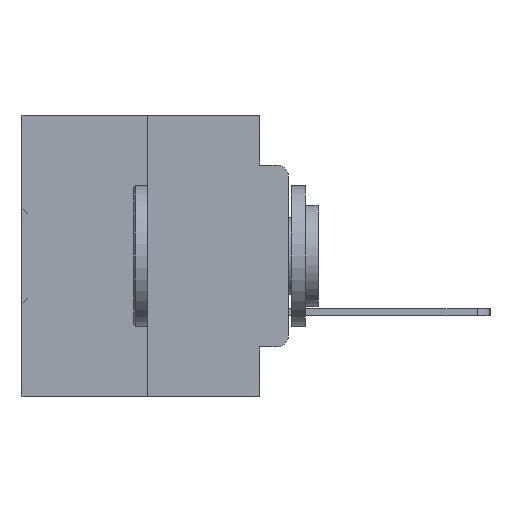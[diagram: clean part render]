
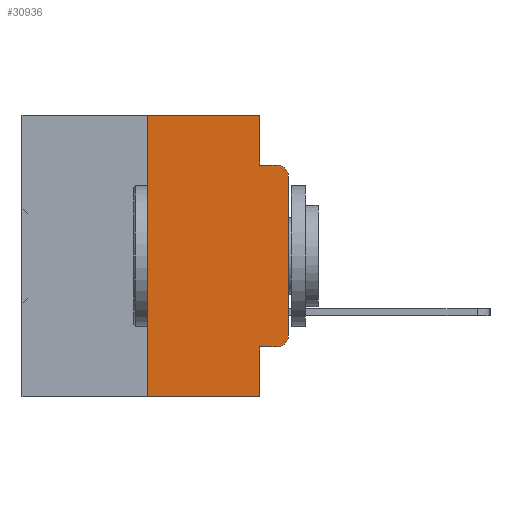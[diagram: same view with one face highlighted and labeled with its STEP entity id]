
A CAD part, left-side view. The second image highlights one B-rep face of the part: STEP entity #30936.
In plain terms, the highlighted planar face has unit normal (-1, 0, 0).
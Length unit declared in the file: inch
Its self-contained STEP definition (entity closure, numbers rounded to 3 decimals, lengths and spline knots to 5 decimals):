
#434 = EDGE_CURVE ( 'NONE', #21544, #3666, #11660, .T. ) ;
#858 = LINE ( 'NONE', #2603, #28845 ) ;
#1403 = DIRECTION ( 'NONE',  ( 0., -1., 0. ) ) ;
#2603 = CARTESIAN_POINT ( 'NONE',  ( 0., 0.051, 0. ) ) ;
#3363 = VECTOR ( 'NONE', #6570, 39.37008 ) ;
#3666 = VERTEX_POINT ( 'NONE', #14622 ) ;
#3934 = CARTESIAN_POINT ( 'NONE',  ( 0., 0.02, -0.4115 ) ) ;
#4176 = ORIENTED_EDGE ( 'NONE', *, *, #11618, .T. ) ;
#4293 = CARTESIAN_POINT ( 'NONE',  ( 0., 0.25, 0. ) ) ;
#4491 = DIRECTION ( 'NONE',  ( 0., 0., 1. ) ) ;
#4858 = DIRECTION ( 'NONE',  ( 0., 0., -1. ) ) ;
#5306 = CARTESIAN_POINT ( 'NONE',  ( 0., 0.051, -0.5 ) ) ;
#6570 = DIRECTION ( 'NONE',  ( 0., 0., 1. ) ) ;
#7183 = LINE ( 'NONE', #12936, #22173 ) ;
#7566 = LINE ( 'NONE', #7788, #21668 ) ;
#7788 = CARTESIAN_POINT ( 'NONE',  ( 0., 0.051, -0.0885 ) ) ;
#7818 = CARTESIAN_POINT ( 'NONE',  ( 0., 0.051, 0. ) ) ;
#8571 = LINE ( 'NONE', #11270, #30840 ) ;
#9204 = VERTEX_POINT ( 'NONE', #5306 ) ;
#9819 = DIRECTION ( 'NONE',  ( -1., 0., 0. ) ) ;
#9824 = EDGE_CURVE ( 'NONE', #34088, #9204, #858, .T. ) ;
#10353 = AXIS2_PLACEMENT_3D ( 'NONE', #26600, #9819, #29366 ) ;
#10611 = DIRECTION ( 'NONE',  ( 0., -1., 0. ) ) ;
#11270 = CARTESIAN_POINT ( 'NONE',  ( 0., 0.051, -0.4115 ) ) ;
#11326 = EDGE_CURVE ( 'NONE', #3666, #15768, #35539, .T. ) ;
#11618 = EDGE_CURVE ( 'NONE', #21544, #9204, #33386, .T. ) ;
#11660 = LINE ( 'NONE', #4293, #3363 ) ;
#11675 = EDGE_CURVE ( 'NONE', #34088, #20534, #8571, .T. ) ;
#12374 = EDGE_CURVE ( 'NONE', #32485, #26978, #7183, .T. ) ;
#12926 = VERTEX_POINT ( 'NONE', #15897 ) ;
#12936 = CARTESIAN_POINT ( 'NONE',  ( 0., 0., 0. ) ) ;
#12945 = DIRECTION ( 'NONE',  ( -1., 0., 0. ) ) ;
#14622 = CARTESIAN_POINT ( 'NONE',  ( 0., 0.25, 0. ) ) ;
#15768 = VERTEX_POINT ( 'NONE', #19610 ) ;
#15897 = CARTESIAN_POINT ( 'NONE',  ( 0., 0.051, -0.0885 ) ) ;
#16616 = CARTESIAN_POINT ( 'NONE',  ( 0., 0., -0.3915 ) ) ;
#17797 = LINE ( 'NONE', #7818, #33356 ) ;
#18198 = CARTESIAN_POINT ( 'NONE',  ( 0., 0.473, 0. ) ) ;
#18888 = CARTESIAN_POINT ( 'NONE',  ( 0., 0.473, 0. ) ) ;
#19427 = CARTESIAN_POINT ( 'NONE',  ( 0., 0.473, -0.5 ) ) ;
#19610 = CARTESIAN_POINT ( 'NONE',  ( 0., 0.051, 0. ) ) ;
#20534 = VERTEX_POINT ( 'NONE', #3934 ) ;
#21140 = EDGE_CURVE ( 'NONE', #20534, #32485, #33394, .T. ) ;
#21544 = VERTEX_POINT ( 'NONE', #30998 ) ;
#21668 = VECTOR ( 'NONE', #10611, 39.37008 ) ;
#21682 = AXIS2_PLACEMENT_3D ( 'NONE', #18888, #21716, #4858 ) ;
#21716 = DIRECTION ( 'NONE',  ( 1., 0., 0. ) ) ;
#21848 = EDGE_CURVE ( 'NONE', #26978, #22989, #25652, .T. ) ;
#22038 = CARTESIAN_POINT ( 'NONE',  ( 0., 0.051, -0.4115 ) ) ;
#22173 = VECTOR ( 'NONE', #4491, 39.37008 ) ;
#22989 = VERTEX_POINT ( 'NONE', #25548 ) ;
#23735 = EDGE_CURVE ( 'NONE', #12926, #22989, #7566, .T. ) ;
#24483 = EDGE_LOOP ( 'NONE', ( #26079, #26947, #35911, #29550, #31238, #24814, #4176, #26537, #34633, #35496 ) ) ;
#24814 = ORIENTED_EDGE ( 'NONE', *, *, #434, .F. ) ;
#25254 = CARTESIAN_POINT ( 'NONE',  ( 0., 0., -0.1085 ) ) ;
#25268 = VECTOR ( 'NONE', #35903, 39.37008 ) ;
#25548 = CARTESIAN_POINT ( 'NONE',  ( 0., 0.02, -0.0885 ) ) ;
#25652 = CIRCLE ( 'NONE', #25857, 0.02 ) ;
#25857 = AXIS2_PLACEMENT_3D ( 'NONE', #29688, #12945, #32399 ) ;
#26079 = ORIENTED_EDGE ( 'NONE', *, *, #12374, .T. ) ;
#26537 = ORIENTED_EDGE ( 'NONE', *, *, #9824, .F. ) ;
#26600 = CARTESIAN_POINT ( 'NONE',  ( 0., 0.02, -0.3915 ) ) ;
#26947 = ORIENTED_EDGE ( 'NONE', *, *, #21848, .T. ) ;
#26978 = VERTEX_POINT ( 'NONE', #25254 ) ;
#27420 = DIRECTION ( 'NONE',  ( 0., 0., -1. ) ) ;
#27801 = DIRECTION ( 'NONE',  ( 0., 0., -1. ) ) ;
#28845 = VECTOR ( 'NONE', #27801, 39.37008 ) ;
#29161 = VECTOR ( 'NONE', #1403, 39.37008 ) ;
#29366 = DIRECTION ( 'NONE',  ( 0., 0., -1. ) ) ;
#29550 = ORIENTED_EDGE ( 'NONE', *, *, #34700, .F. ) ;
#29688 = CARTESIAN_POINT ( 'NONE',  ( 0., 0.02, -0.1085 ) ) ;
#30009 = FACE_OUTER_BOUND ( 'NONE', #24483, .T. ) ;
#30788 = DIRECTION ( 'NONE',  ( 0., -1., 0. ) ) ;
#30840 = VECTOR ( 'NONE', #30788, 39.37008 ) ;
#30936 = ADVANCED_FACE ( 'NONE', ( #30009 ), #35382, .F. ) ;
#30998 = CARTESIAN_POINT ( 'NONE',  ( 0., 0.25, -0.5 ) ) ;
#31238 = ORIENTED_EDGE ( 'NONE', *, *, #11326, .F. ) ;
#32399 = DIRECTION ( 'NONE',  ( 0., 0., -1. ) ) ;
#32485 = VERTEX_POINT ( 'NONE', #16616 ) ;
#33356 = VECTOR ( 'NONE', #27420, 39.37008 ) ;
#33386 = LINE ( 'NONE', #19427, #25268 ) ;
#33394 = CIRCLE ( 'NONE', #10353, 0.02 ) ;
#34088 = VERTEX_POINT ( 'NONE', #22038 ) ;
#34633 = ORIENTED_EDGE ( 'NONE', *, *, #11675, .T. ) ;
#34700 = EDGE_CURVE ( 'NONE', #15768, #12926, #17797, .T. ) ;
#35382 = PLANE ( 'NONE',  #21682 ) ;
#35496 = ORIENTED_EDGE ( 'NONE', *, *, #21140, .T. ) ;
#35539 = LINE ( 'NONE', #18198, #29161 ) ;
#35903 = DIRECTION ( 'NONE',  ( 0., -1., 0. ) ) ;
#35911 = ORIENTED_EDGE ( 'NONE', *, *, #23735, .F. ) ;
